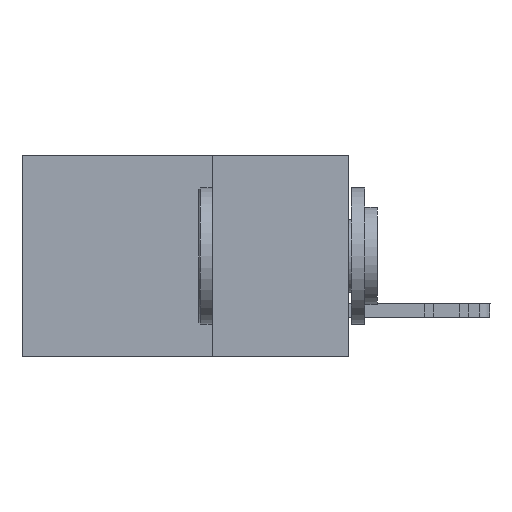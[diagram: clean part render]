
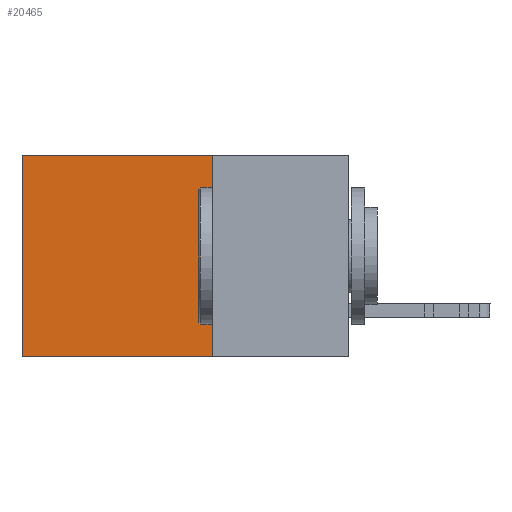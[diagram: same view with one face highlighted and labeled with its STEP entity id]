
A CAD part, left-side view. The second image highlights one B-rep face of the part: STEP entity #20465.
In plain terms, the highlighted planar face has unit normal (-1, 0, 0).
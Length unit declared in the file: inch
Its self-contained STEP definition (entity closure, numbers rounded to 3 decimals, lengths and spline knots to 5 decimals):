
#989 = VECTOR ( 'NONE', #21714, 39.37008 ) ;
#2098 = CARTESIAN_POINT ( 'NONE',  ( 0.2615, 0.25, -0.37 ) ) ;
#2203 = DIRECTION ( 'NONE',  ( 0., 1., 0. ) ) ;
#3155 = VERTEX_POINT ( 'NONE', #10421 ) ;
#3810 = VECTOR ( 'NONE', #10858, 39.37008 ) ;
#4047 = CARTESIAN_POINT ( 'NONE',  ( 0.2615, 0.25, -0.37 ) ) ;
#4049 = DIRECTION ( 'NONE',  ( 1., 0., 0. ) ) ;
#4161 = CARTESIAN_POINT ( 'NONE',  ( 0.2615, 0.25, -0.37 ) ) ;
#4342 = CARTESIAN_POINT ( 'NONE',  ( 0.2615, 0.25, 0. ) ) ;
#5472 = EDGE_CURVE ( 'NONE', #14963, #21051, #11179, .T. ) ;
#5687 = LINE ( 'NONE', #4047, #3810 ) ;
#6091 = ORIENTED_EDGE ( 'NONE', *, *, #7584, .T. ) ;
#6297 = VECTOR ( 'NONE', #18939, 39.37008 ) ;
#7314 = AXIS2_PLACEMENT_3D ( 'NONE', #4161, #4049, #18241 ) ;
#7584 = EDGE_CURVE ( 'NONE', #14963, #3155, #22307, .T. ) ;
#8063 = CARTESIAN_POINT ( 'NONE',  ( 0.2615, 0.6, -0.37 ) ) ;
#8573 = EDGE_CURVE ( 'NONE', #3155, #14565, #16823, .T. ) ;
#10421 = CARTESIAN_POINT ( 'NONE',  ( 0.2615, 0.6, 0. ) ) ;
#10858 = DIRECTION ( 'NONE',  ( 0., 1., 0. ) ) ;
#11055 = ORIENTED_EDGE ( 'NONE', *, *, #14883, .F. ) ;
#11179 = LINE ( 'NONE', #2098, #989 ) ;
#11744 = ORIENTED_EDGE ( 'NONE', *, *, #5472, .F. ) ;
#13411 = EDGE_LOOP ( 'NONE', ( #22545, #11055, #11744, #6091 ) ) ;
#14240 = VECTOR ( 'NONE', #2203, 39.37008 ) ;
#14565 = VERTEX_POINT ( 'NONE', #15505 ) ;
#14774 = CARTESIAN_POINT ( 'NONE',  ( 0.2615, 0.25, 0. ) ) ;
#14883 = EDGE_CURVE ( 'NONE', #21051, #14565, #5687, .T. ) ;
#14963 = VERTEX_POINT ( 'NONE', #14774 ) ;
#15505 = CARTESIAN_POINT ( 'NONE',  ( 0.2615, 0.6, -0.37 ) ) ;
#16583 = FACE_OUTER_BOUND ( 'NONE', #13411, .T. ) ;
#16823 = LINE ( 'NONE', #8063, #6297 ) ;
#18241 = DIRECTION ( 'NONE',  ( 0., 0., -1. ) ) ;
#18897 = CARTESIAN_POINT ( 'NONE',  ( 0.2615, 0.25, -0.37 ) ) ;
#18939 = DIRECTION ( 'NONE',  ( 0., 0., -1. ) ) ;
#20217 = PLANE ( 'NONE',  #7314 ) ;
#20465 = ADVANCED_FACE ( 'NONE', ( #16583 ), #20217, .F. ) ;
#21051 = VERTEX_POINT ( 'NONE', #18897 ) ;
#21714 = DIRECTION ( 'NONE',  ( 0., 0., -1. ) ) ;
#22307 = LINE ( 'NONE', #4342, #14240 ) ;
#22545 = ORIENTED_EDGE ( 'NONE', *, *, #8573, .T. ) ;
